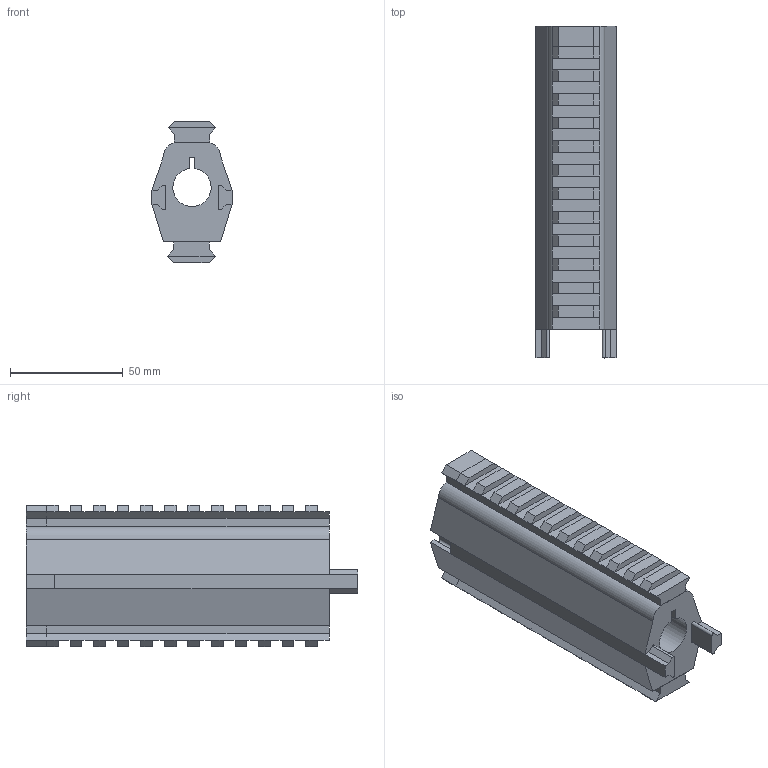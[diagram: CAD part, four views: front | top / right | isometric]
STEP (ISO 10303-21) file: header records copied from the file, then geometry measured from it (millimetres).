
FILE_DESCRIPTION(/* description */ (''),/* implementation_level */ '2;1');
FILE_NAME(/* name */ 'HRR PRA - 16in 5.3in Extension v2.step',/* time_stamp */ '2019-12-24T23:46:39-05:00',/* author */ (''),/* organization */ (''),/* preprocessor_version */ 'ST-DEVELOPER v18',/* originating_system */ 'Autodesk Translation Framework v8.12.0.6',/* authorisation */ '');
FILE_SCHEMA (('AUTOMOTIVE_DESIGN { 1 0 10303 214 3 1 1 }'));
Length unit declared in the file: millimetre
Products named in the file (1): HRR PRA - 16in 5.3in Extension
Bounding box: 35.56 x 147.32 x 62.84 mm (x, y, z)
Volume: 183879.6 mm3; surface area: 48380.6 mm2
Topology: 5 solids, 5 shells, 226 faces, 596 edges, 380 vertices
Faces by surface type: plane 215, cylinder 11
Entity records: 6819 total; most frequent: CARTESIAN_POINT 1203, ORIENTED_EDGE 1192, DIRECTION 1072, EDGE_CURVE 596, LINE 574, VECTOR 574, VERTEX_POINT 380, AXIS2_PLACEMENT_3D 249
